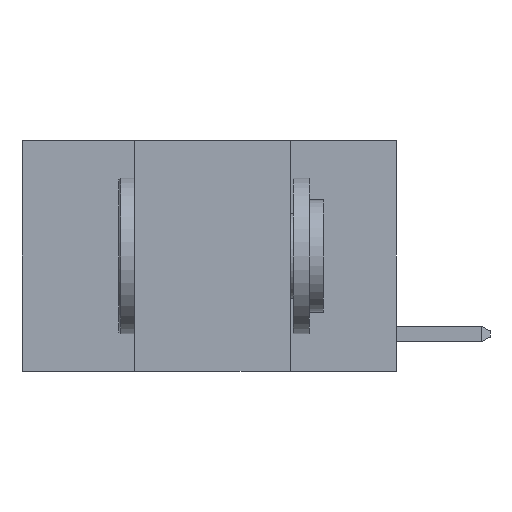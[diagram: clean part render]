
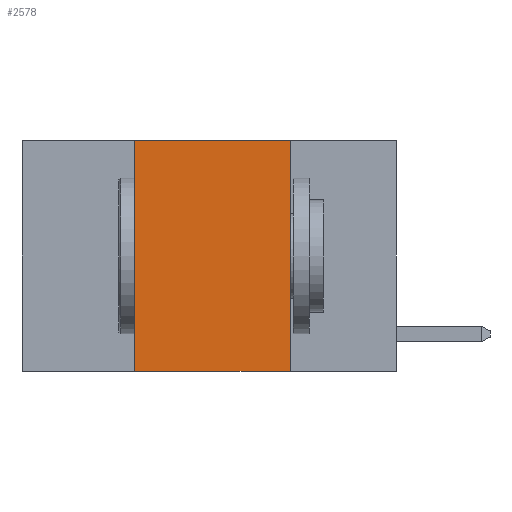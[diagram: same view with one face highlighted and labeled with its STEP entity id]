
A CAD part, left-side view. The second image highlights one B-rep face of the part: STEP entity #2578.
In plain terms, the highlighted planar face has unit normal (-1, 0, 0).
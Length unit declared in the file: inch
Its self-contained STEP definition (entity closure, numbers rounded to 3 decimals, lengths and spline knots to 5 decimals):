
#72 = CARTESIAN_POINT ( 'NONE',  ( 0., 0.6, -0.37 ) ) ;
#453 = LINE ( 'NONE', #72, #5190 ) ;
#861 = CARTESIAN_POINT ( 'NONE',  ( 0., 0.6, 0. ) ) ;
#912 = EDGE_CURVE ( 'NONE', #9387, #8268, #11604, .T. ) ;
#950 = EDGE_CURVE ( 'NONE', #1776, #6573, #6094, .T. ) ;
#987 = CARTESIAN_POINT ( 'NONE',  ( 0., 0.17, -0.37 ) ) ;
#1101 = DIRECTION ( 'NONE',  ( 0., -1., 0. ) ) ;
#1151 = EDGE_CURVE ( 'NONE', #8268, #1776, #8618, .T. ) ;
#1776 = VERTEX_POINT ( 'NONE', #11359 ) ;
#1911 = AXIS2_PLACEMENT_3D ( 'NONE', #3606, #9940, #4561 ) ;
#2030 = VECTOR ( 'NONE', #2602, 39.37008 ) ;
#2245 = ORIENTED_EDGE ( 'NONE', *, *, #950, .F. ) ;
#2526 = CARTESIAN_POINT ( 'NONE',  ( 0., 0.42, 0. ) ) ;
#2578 = ADVANCED_FACE ( 'NONE', ( #10853 ), #9073, .F. ) ;
#2602 = DIRECTION ( 'NONE',  ( 0., 0., 1. ) ) ;
#3599 = VECTOR ( 'NONE', #9712, 39.37008 ) ;
#3606 = CARTESIAN_POINT ( 'NONE',  ( 0., 0.6, 0. ) ) ;
#3831 = EDGE_LOOP ( 'NONE', ( #2245, #4705, #7107, #5023 ) ) ;
#4561 = DIRECTION ( 'NONE',  ( 0., 0., -1. ) ) ;
#4705 = ORIENTED_EDGE ( 'NONE', *, *, #1151, .F. ) ;
#5023 = ORIENTED_EDGE ( 'NONE', *, *, #7435, .T. ) ;
#5190 = VECTOR ( 'NONE', #1101, 39.37008 ) ;
#6094 = LINE ( 'NONE', #9238, #3599 ) ;
#6573 = VERTEX_POINT ( 'NONE', #987 ) ;
#7107 = ORIENTED_EDGE ( 'NONE', *, *, #912, .F. ) ;
#7353 = DIRECTION ( 'NONE',  ( 0., -1., 0. ) ) ;
#7435 = EDGE_CURVE ( 'NONE', #9387, #6573, #453, .T. ) ;
#7490 = CARTESIAN_POINT ( 'NONE',  ( 0., 0.42, 0. ) ) ;
#8028 = VECTOR ( 'NONE', #7353, 39.37008 ) ;
#8268 = VERTEX_POINT ( 'NONE', #7490 ) ;
#8618 = LINE ( 'NONE', #861, #8028 ) ;
#9073 = PLANE ( 'NONE',  #1911 ) ;
#9238 = CARTESIAN_POINT ( 'NONE',  ( 0., 0.17, 0. ) ) ;
#9387 = VERTEX_POINT ( 'NONE', #10775 ) ;
#9712 = DIRECTION ( 'NONE',  ( 0., 0., -1. ) ) ;
#9940 = DIRECTION ( 'NONE',  ( 1., 0., 0. ) ) ;
#10775 = CARTESIAN_POINT ( 'NONE',  ( 0., 0.42, -0.37 ) ) ;
#10853 = FACE_OUTER_BOUND ( 'NONE', #3831, .T. ) ;
#11359 = CARTESIAN_POINT ( 'NONE',  ( 0., 0.17, 0. ) ) ;
#11604 = LINE ( 'NONE', #2526, #2030 ) ;
